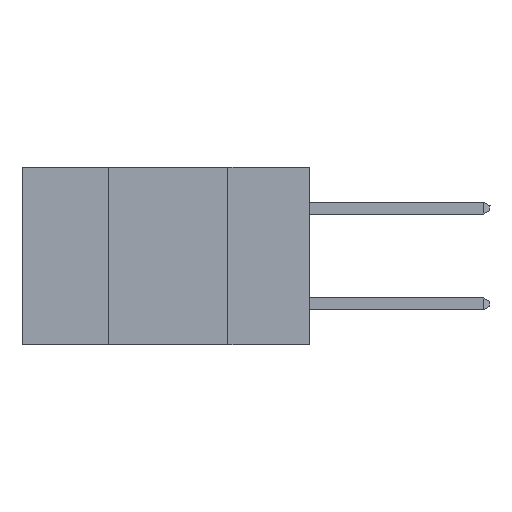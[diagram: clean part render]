
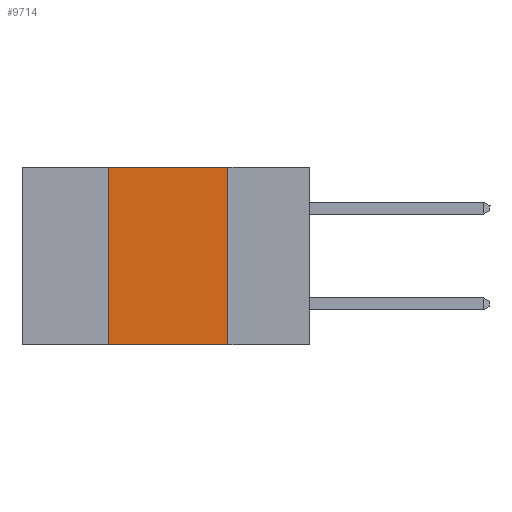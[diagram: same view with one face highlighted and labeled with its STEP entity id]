
A CAD part, left-side view. The second image highlights one B-rep face of the part: STEP entity #9714.
In plain terms, the highlighted planar face has unit normal (-1, 0, 0).
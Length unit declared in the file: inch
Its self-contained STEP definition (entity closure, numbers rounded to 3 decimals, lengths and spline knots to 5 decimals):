
#513 = CARTESIAN_POINT ( 'NONE',  ( 0., 0.42, -0.37 ) ) ;
#953 = ORIENTED_EDGE ( 'NONE', *, *, #2181, .F. ) ;
#1386 = VERTEX_POINT ( 'NONE', #513 ) ;
#1477 = DIRECTION ( 'NONE',  ( 0., -1., 0. ) ) ;
#1544 = AXIS2_PLACEMENT_3D ( 'NONE', #2233, #9644, #3386 ) ;
#1658 = CARTESIAN_POINT ( 'NONE',  ( 0., 0.42, 0. ) ) ;
#1821 = CARTESIAN_POINT ( 'NONE',  ( 0., 0.17, 0. ) ) ;
#2181 = EDGE_CURVE ( 'NONE', #1386, #12203, #3007, .T. ) ;
#2233 = CARTESIAN_POINT ( 'NONE',  ( 0., 0.6, 0. ) ) ;
#2262 = EDGE_CURVE ( 'NONE', #12521, #9322, #12365, .T. ) ;
#2412 = LINE ( 'NONE', #10932, #4961 ) ;
#2423 = CARTESIAN_POINT ( 'NONE',  ( 0., 0.17, -0.37 ) ) ;
#2466 = EDGE_LOOP ( 'NONE', ( #10303, #8964, #953, #6649 ) ) ;
#2628 = VECTOR ( 'NONE', #12910, 39.37008 ) ;
#2872 = VECTOR ( 'NONE', #10630, 39.37008 ) ;
#3007 = LINE ( 'NONE', #1658, #2628 ) ;
#3367 = CARTESIAN_POINT ( 'NONE',  ( 0., 0.6, -0.37 ) ) ;
#3386 = DIRECTION ( 'NONE',  ( 0., 0., -1. ) ) ;
#4961 = VECTOR ( 'NONE', #1477, 39.37008 ) ;
#5927 = CARTESIAN_POINT ( 'NONE',  ( 0., 0.17, 0. ) ) ;
#6649 = ORIENTED_EDGE ( 'NONE', *, *, #10460, .T. ) ;
#6906 = DIRECTION ( 'NONE',  ( 0., 0., -1. ) ) ;
#7033 = EDGE_CURVE ( 'NONE', #12203, #12521, #2412, .T. ) ;
#8964 = ORIENTED_EDGE ( 'NONE', *, *, #7033, .F. ) ;
#9322 = VERTEX_POINT ( 'NONE', #2423 ) ;
#9457 = CARTESIAN_POINT ( 'NONE',  ( 0., 0.42, 0. ) ) ;
#9644 = DIRECTION ( 'NONE',  ( 1., 0., 0. ) ) ;
#9714 = ADVANCED_FACE ( 'NONE', ( #12131 ), #13466, .F. ) ;
#9728 = VECTOR ( 'NONE', #6906, 39.37008 ) ;
#10303 = ORIENTED_EDGE ( 'NONE', *, *, #2262, .F. ) ;
#10460 = EDGE_CURVE ( 'NONE', #1386, #9322, #13120, .T. ) ;
#10630 = DIRECTION ( 'NONE',  ( 0., -1., 0. ) ) ;
#10932 = CARTESIAN_POINT ( 'NONE',  ( 0., 0.6, 0. ) ) ;
#12131 = FACE_OUTER_BOUND ( 'NONE', #2466, .T. ) ;
#12203 = VERTEX_POINT ( 'NONE', #9457 ) ;
#12365 = LINE ( 'NONE', #1821, #9728 ) ;
#12521 = VERTEX_POINT ( 'NONE', #5927 ) ;
#12910 = DIRECTION ( 'NONE',  ( 0., 0., 1. ) ) ;
#13120 = LINE ( 'NONE', #3367, #2872 ) ;
#13466 = PLANE ( 'NONE',  #1544 ) ;
